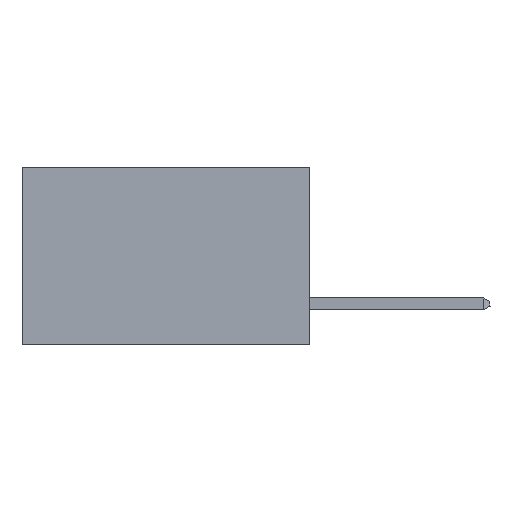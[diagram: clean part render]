
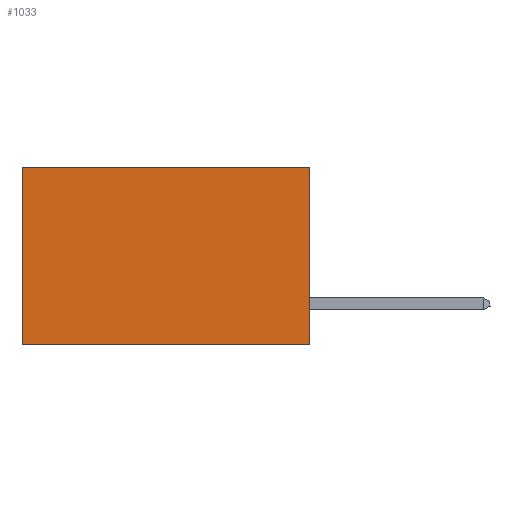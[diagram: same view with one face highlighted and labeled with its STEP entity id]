
A CAD part, left-side view. The second image highlights one B-rep face of the part: STEP entity #1033.
In plain terms, the highlighted planar face has unit normal (-1, 0, 0).
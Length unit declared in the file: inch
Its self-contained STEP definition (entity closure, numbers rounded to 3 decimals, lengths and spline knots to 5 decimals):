
#1033 = ADVANCED_FACE ( 'NONE', ( #14499 ), #15255, .F. ) ;
#1098 = EDGE_CURVE ( 'NONE', #17529, #11076, #10850, .T. ) ;
#1465 = DIRECTION ( 'NONE',  ( 0., 0., -1. ) ) ;
#1633 = VERTEX_POINT ( 'NONE', #5928 ) ;
#1795 = CARTESIAN_POINT ( 'NONE',  ( 0.2875, 0., 0. ) ) ;
#2320 = DIRECTION ( 'NONE',  ( 0., 1., 0. ) ) ;
#3608 = CARTESIAN_POINT ( 'NONE',  ( 0.2875, 0.6, 0. ) ) ;
#4451 = LINE ( 'NONE', #17266, #4678 ) ;
#4678 = VECTOR ( 'NONE', #2320, 39.37008 ) ;
#4728 = CARTESIAN_POINT ( 'NONE',  ( 0.2875, 0., 0. ) ) ;
#5928 = CARTESIAN_POINT ( 'NONE',  ( 0.2875, 0., -0.37 ) ) ;
#6318 = ORIENTED_EDGE ( 'NONE', *, *, #15288, .F. ) ;
#6489 = CARTESIAN_POINT ( 'NONE',  ( 0.2875, 0., 0. ) ) ;
#6967 = CARTESIAN_POINT ( 'NONE',  ( 0.2875, 0., 0. ) ) ;
#7651 = DIRECTION ( 'NONE',  ( 0., 0., -1. ) ) ;
#7774 = VECTOR ( 'NONE', #11314, 39.37008 ) ;
#7988 = ORIENTED_EDGE ( 'NONE', *, *, #11380, .T. ) ;
#10673 = VECTOR ( 'NONE', #7651, 39.37008 ) ;
#10850 = LINE ( 'NONE', #1795, #7774 ) ;
#11076 = VERTEX_POINT ( 'NONE', #14340 ) ;
#11314 = DIRECTION ( 'NONE',  ( 0., 1., 0. ) ) ;
#11380 = EDGE_CURVE ( 'NONE', #11076, #12815, #13038, .T. ) ;
#12815 = VERTEX_POINT ( 'NONE', #17107 ) ;
#13038 = LINE ( 'NONE', #3608, #10673 ) ;
#13675 = EDGE_LOOP ( 'NONE', ( #7988, #6318, #13786, #16375 ) ) ;
#13786 = ORIENTED_EDGE ( 'NONE', *, *, #16117, .F. ) ;
#14340 = CARTESIAN_POINT ( 'NONE',  ( 0.2875, 0.6, 0. ) ) ;
#14341 = VECTOR ( 'NONE', #14557, 39.37008 ) ;
#14499 = FACE_OUTER_BOUND ( 'NONE', #13675, .T. ) ;
#14557 = DIRECTION ( 'NONE',  ( 0., 0., -1. ) ) ;
#14833 = AXIS2_PLACEMENT_3D ( 'NONE', #6967, #17756, #1465 ) ;
#15255 = PLANE ( 'NONE',  #14833 ) ;
#15288 = EDGE_CURVE ( 'NONE', #1633, #12815, #4451, .T. ) ;
#16117 = EDGE_CURVE ( 'NONE', #17529, #1633, #17752, .T. ) ;
#16375 = ORIENTED_EDGE ( 'NONE', *, *, #1098, .T. ) ;
#17107 = CARTESIAN_POINT ( 'NONE',  ( 0.2875, 0.6, -0.37 ) ) ;
#17266 = CARTESIAN_POINT ( 'NONE',  ( 0.2875, 0., -0.37 ) ) ;
#17529 = VERTEX_POINT ( 'NONE', #4728 ) ;
#17752 = LINE ( 'NONE', #6489, #14341 ) ;
#17756 = DIRECTION ( 'NONE',  ( 1., 0., 0. ) ) ;
